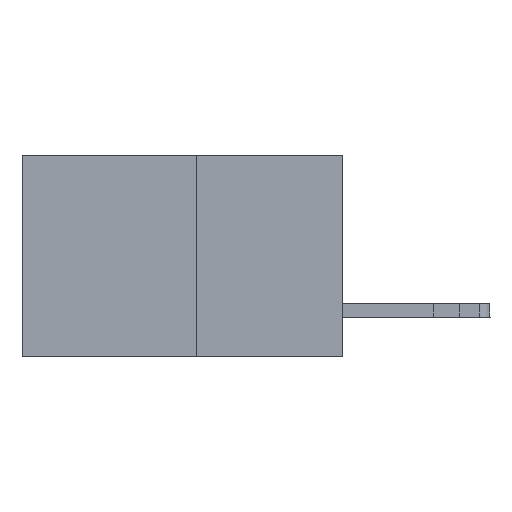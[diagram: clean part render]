
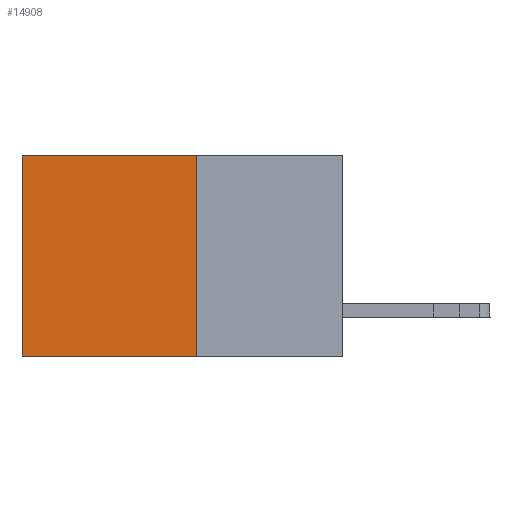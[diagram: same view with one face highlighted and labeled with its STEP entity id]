
A CAD part, left-side view. The second image highlights one B-rep face of the part: STEP entity #14908.
In plain terms, the highlighted planar face has unit normal (-1, 0, 0).
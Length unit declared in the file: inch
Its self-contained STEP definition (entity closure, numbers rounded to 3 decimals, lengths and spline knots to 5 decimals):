
#1165 = LINE ( 'NONE', #5767, #2926 ) ;
#1586 = DIRECTION ( 'NONE',  ( 0., 0., -1. ) ) ;
#2386 = EDGE_CURVE ( 'NONE', #14670, #18045, #1165, .T. ) ;
#2926 = VECTOR ( 'NONE', #14540, 39.37008 ) ;
#3490 = PLANE ( 'NONE',  #17696 ) ;
#3562 = ORIENTED_EDGE ( 'NONE', *, *, #15950, .T. ) ;
#3585 = CARTESIAN_POINT ( 'NONE',  ( 0.277, 0.27, -0.37 ) ) ;
#3994 = CARTESIAN_POINT ( 'NONE',  ( 0.277, 0.27, 0. ) ) ;
#4678 = CARTESIAN_POINT ( 'NONE',  ( 0.277, 0.59, 0. ) ) ;
#5767 = CARTESIAN_POINT ( 'NONE',  ( 0.277, 0.27, -0.37 ) ) ;
#5848 = VERTEX_POINT ( 'NONE', #4678 ) ;
#6300 = ORIENTED_EDGE ( 'NONE', *, *, #2386, .F. ) ;
#6585 = FACE_OUTER_BOUND ( 'NONE', #8837, .T. ) ;
#7543 = DIRECTION ( 'NONE',  ( 0., 0., -1. ) ) ;
#8477 = ORIENTED_EDGE ( 'NONE', *, *, #13570, .T. ) ;
#8837 = EDGE_LOOP ( 'NONE', ( #3562, #6300, #9683, #8477 ) ) ;
#9065 = VECTOR ( 'NONE', #16785, 39.37008 ) ;
#9370 = CARTESIAN_POINT ( 'NONE',  ( 0.277, 0.59, -0.37 ) ) ;
#9566 = DIRECTION ( 'NONE',  ( 1., 0., 0. ) ) ;
#9683 = ORIENTED_EDGE ( 'NONE', *, *, #11276, .F. ) ;
#10271 = VECTOR ( 'NONE', #1586, 39.37008 ) ;
#10516 = CARTESIAN_POINT ( 'NONE',  ( 0.277, 0.27, 0. ) ) ;
#10622 = CARTESIAN_POINT ( 'NONE',  ( 0.277, 0.27, -0.37 ) ) ;
#10716 = LINE ( 'NONE', #10516, #9065 ) ;
#11276 = EDGE_CURVE ( 'NONE', #19658, #14670, #16595, .T. ) ;
#11907 = VECTOR ( 'NONE', #7543, 39.37008 ) ;
#12257 = LINE ( 'NONE', #9370, #10271 ) ;
#13036 = CARTESIAN_POINT ( 'NONE',  ( 0.277, 0.59, -0.37 ) ) ;
#13352 = CARTESIAN_POINT ( 'NONE',  ( 0.277, 0.27, -0.37 ) ) ;
#13570 = EDGE_CURVE ( 'NONE', #19658, #5848, #10716, .T. ) ;
#14540 = DIRECTION ( 'NONE',  ( 0., 1., 0. ) ) ;
#14670 = VERTEX_POINT ( 'NONE', #13352 ) ;
#14908 = ADVANCED_FACE ( 'NONE', ( #6585 ), #3490, .F. ) ;
#15950 = EDGE_CURVE ( 'NONE', #5848, #18045, #12257, .T. ) ;
#16595 = LINE ( 'NONE', #10622, #11907 ) ;
#16785 = DIRECTION ( 'NONE',  ( 0., 1., 0. ) ) ;
#17696 = AXIS2_PLACEMENT_3D ( 'NONE', #3585, #9566, #18451 ) ;
#18045 = VERTEX_POINT ( 'NONE', #13036 ) ;
#18451 = DIRECTION ( 'NONE',  ( 0., 0., -1. ) ) ;
#19658 = VERTEX_POINT ( 'NONE', #3994 ) ;
